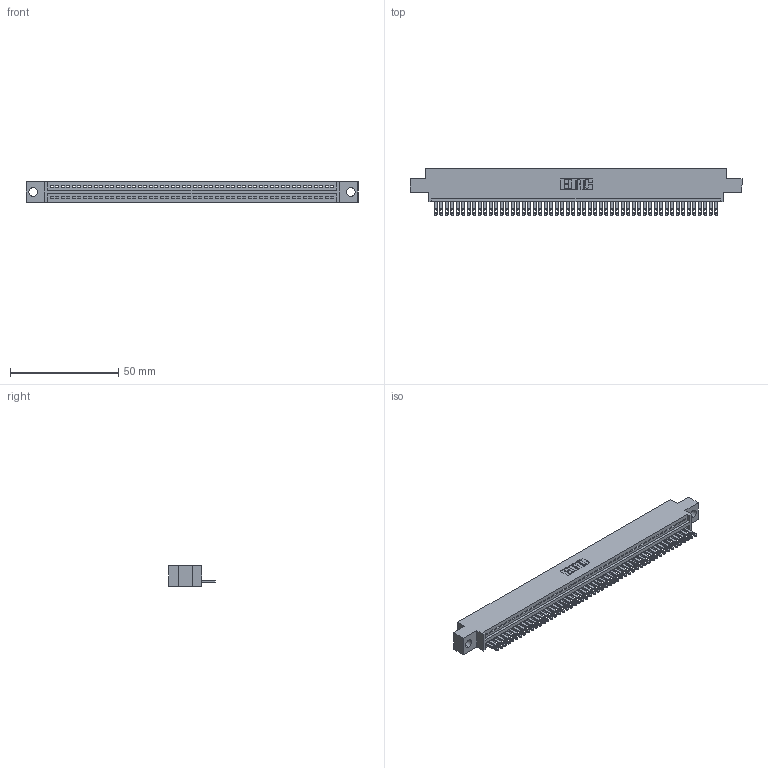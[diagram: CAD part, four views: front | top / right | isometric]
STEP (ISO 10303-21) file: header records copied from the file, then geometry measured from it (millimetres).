
FILE_DESCRIPTION (( 'STEP AP203' ), '1' );
FILE_NAME ('345-052-500-604.STEP', '2018-09-22T19:21:55', ( '' ), ( '' ), 'SwSTEP 2.0', 'SolidWorks 2016', '' );
FILE_SCHEMA (( 'CONFIG_CONTROL_DESIGN' ));
Length unit declared in the file: inch
Products named in the file (3): 345 Part_0.170 Offset - 0.156 Dia-TH; 345-292-001_345-293-100; 345-052-500-604
Assembly tree (53 placements, depth 2):
  345-052-500-604
    345 Part_0.170 Offset - 0.156 Dia-TH
    345-292-001_345-293-100  x52
Bounding box: 153.29 x 21.51 x 9.4 mm (x, y, z)
Volume: 14472.4 mm3; surface area: 19420.5 mm2
Topology: 53 solids, 53 shells, 2938 faces, 9089 edges, 6058 vertices
Faces by surface type: plane 1852, cylinder 1086
Entity records: 37855 total; most frequent: CARTESIAN_POINT 6564, ORIENTED_EDGE 6550, DIRECTION 5719, EDGE_CURVE 3275, LINE 2931, VECTOR 2931, VERTEX_POINT 2182, AXIS2_PLACEMENT_3D 1394
